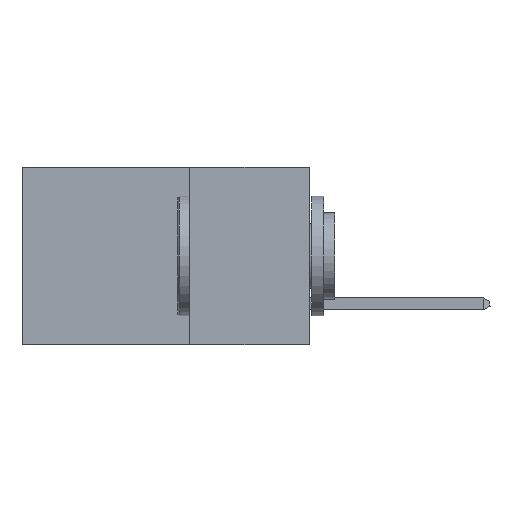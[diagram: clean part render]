
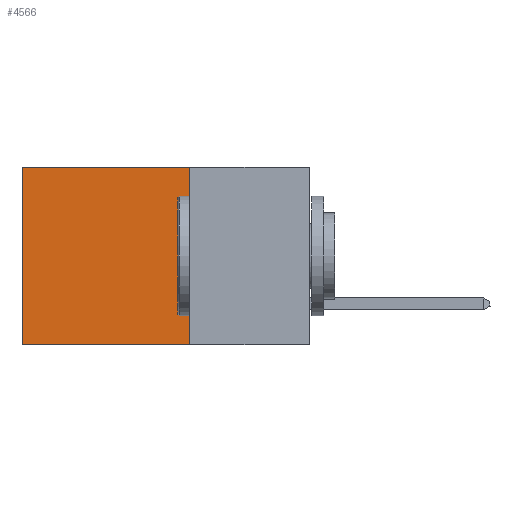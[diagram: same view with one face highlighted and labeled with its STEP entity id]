
A CAD part, left-side view. The second image highlights one B-rep face of the part: STEP entity #4566.
In plain terms, the highlighted planar face has unit normal (-1, 0, 0).
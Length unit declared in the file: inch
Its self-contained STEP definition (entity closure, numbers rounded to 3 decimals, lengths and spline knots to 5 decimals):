
#110 = EDGE_LOOP ( 'NONE', ( #5572, #8641, #7632, #7055 ) ) ;
#621 = CARTESIAN_POINT ( 'NONE',  ( 0.2875, 0.25, 0. ) ) ;
#1164 = FACE_OUTER_BOUND ( 'NONE', #110, .T. ) ;
#1431 = DIRECTION ( 'NONE',  ( 1., 0., 0. ) ) ;
#1634 = AXIS2_PLACEMENT_3D ( 'NONE', #621, #1431, #6403 ) ;
#2501 = DIRECTION ( 'NONE',  ( 0., 0., -1. ) ) ;
#3468 = VECTOR ( 'NONE', #8665, 39.37008 ) ;
#3618 = VERTEX_POINT ( 'NONE', #4651 ) ;
#3706 = CARTESIAN_POINT ( 'NONE',  ( 0.2875, 0.25, 0. ) ) ;
#3783 = PLANE ( 'NONE',  #1634 ) ;
#3806 = LINE ( 'NONE', #6700, #9346 ) ;
#4388 = EDGE_CURVE ( 'NONE', #5070, #3618, #5243, .T. ) ;
#4566 = ADVANCED_FACE ( 'NONE', ( #1164 ), #3783, .F. ) ;
#4612 = CARTESIAN_POINT ( 'NONE',  ( 0.2875, 0.25, 0. ) ) ;
#4651 = CARTESIAN_POINT ( 'NONE',  ( 0.2875, 0.6, -0.37 ) ) ;
#4872 = EDGE_CURVE ( 'NONE', #6844, #7214, #9534, .T. ) ;
#4897 = LINE ( 'NONE', #4612, #6954 ) ;
#5070 = VERTEX_POINT ( 'NONE', #8451 ) ;
#5160 = VECTOR ( 'NONE', #6193, 39.37008 ) ;
#5243 = LINE ( 'NONE', #6935, #3468 ) ;
#5572 = ORIENTED_EDGE ( 'NONE', *, *, #7105, .T. ) ;
#6193 = DIRECTION ( 'NONE',  ( 0., 1., 0. ) ) ;
#6403 = DIRECTION ( 'NONE',  ( 0., 0., -1. ) ) ;
#6700 = CARTESIAN_POINT ( 'NONE',  ( 0.2875, 0.6, 0. ) ) ;
#6844 = VERTEX_POINT ( 'NONE', #3706 ) ;
#6935 = CARTESIAN_POINT ( 'NONE',  ( 0.2875, 0.25, -0.37 ) ) ;
#6954 = VECTOR ( 'NONE', #9574, 39.37008 ) ;
#7055 = ORIENTED_EDGE ( 'NONE', *, *, #4872, .T. ) ;
#7105 = EDGE_CURVE ( 'NONE', #7214, #3618, #3806, .T. ) ;
#7123 = CARTESIAN_POINT ( 'NONE',  ( 0.2875, 0.25, 0. ) ) ;
#7214 = VERTEX_POINT ( 'NONE', #7731 ) ;
#7632 = ORIENTED_EDGE ( 'NONE', *, *, #9566, .F. ) ;
#7731 = CARTESIAN_POINT ( 'NONE',  ( 0.2875, 0.6, 0. ) ) ;
#8451 = CARTESIAN_POINT ( 'NONE',  ( 0.2875, 0.25, -0.37 ) ) ;
#8641 = ORIENTED_EDGE ( 'NONE', *, *, #4388, .F. ) ;
#8665 = DIRECTION ( 'NONE',  ( 0., 1., 0. ) ) ;
#9346 = VECTOR ( 'NONE', #2501, 39.37008 ) ;
#9534 = LINE ( 'NONE', #7123, #5160 ) ;
#9566 = EDGE_CURVE ( 'NONE', #6844, #5070, #4897, .T. ) ;
#9574 = DIRECTION ( 'NONE',  ( 0., 0., -1. ) ) ;
